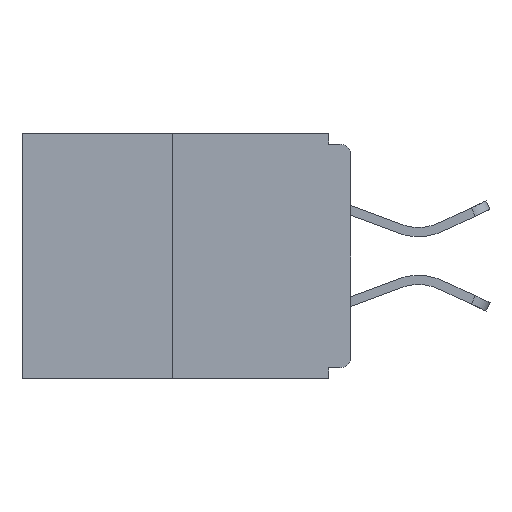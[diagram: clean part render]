
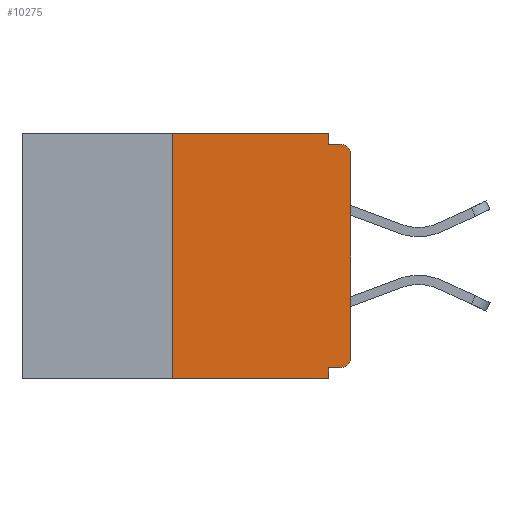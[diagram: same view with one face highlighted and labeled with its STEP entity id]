
A CAD part, left-side view. The second image highlights one B-rep face of the part: STEP entity #10275.
In plain terms, the highlighted planar face has unit normal (-1, 0, 0).
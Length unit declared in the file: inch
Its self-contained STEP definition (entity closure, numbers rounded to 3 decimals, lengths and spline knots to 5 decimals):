
#341 = VECTOR ( 'NONE', #5131, 39.37008 ) ;
#343 = VERTEX_POINT ( 'NONE', #4342 ) ;
#384 = LINE ( 'NONE', #3986, #11502 ) ;
#429 = LINE ( 'NONE', #2580, #6251 ) ;
#442 = CIRCLE ( 'NONE', #6177, 0.015 ) ;
#459 = LINE ( 'NONE', #3136, #7637 ) ;
#1343 = FACE_OUTER_BOUND ( 'NONE', #12251, .T. ) ;
#1357 = CARTESIAN_POINT ( 'NONE',  ( 0., 0.46, -0.343 ) ) ;
#1565 = DIRECTION ( 'NONE',  ( 0., 0., -1. ) ) ;
#1659 = VERTEX_POINT ( 'NONE', #4040 ) ;
#1890 = DIRECTION ( 'NONE',  ( 0., 0., -1. ) ) ;
#2443 = CARTESIAN_POINT ( 'NONE',  ( 0., 0.031, -0.015 ) ) ;
#2580 = CARTESIAN_POINT ( 'NONE',  ( 0., 0., 0. ) ) ;
#2655 = ORIENTED_EDGE ( 'NONE', *, *, #3611, .F. ) ;
#2685 = CARTESIAN_POINT ( 'NONE',  ( 0., 0.031, 0. ) ) ;
#2818 = CARTESIAN_POINT ( 'NONE',  ( 0., 0.015, -0.328 ) ) ;
#3136 = CARTESIAN_POINT ( 'NONE',  ( 0., 0.031, -0.343 ) ) ;
#3190 = VERTEX_POINT ( 'NONE', #12193 ) ;
#3315 = LINE ( 'NONE', #2685, #12921 ) ;
#3611 = EDGE_CURVE ( 'NONE', #18052, #10127, #8825, .T. ) ;
#3906 = DIRECTION ( 'NONE',  ( 0., 1., 0. ) ) ;
#3986 = CARTESIAN_POINT ( 'NONE',  ( 0., 0., -0.015 ) ) ;
#4040 = CARTESIAN_POINT ( 'NONE',  ( 0., 0.015, -0.015 ) ) ;
#4149 = CARTESIAN_POINT ( 'NONE',  ( 0., 0., -0.03 ) ) ;
#4192 = DIRECTION ( 'NONE',  ( -1., 0., 0. ) ) ;
#4341 = DIRECTION ( 'NONE',  ( 0., -1., 0. ) ) ;
#4342 = CARTESIAN_POINT ( 'NONE',  ( 0., 0., -0.313 ) ) ;
#4604 = VERTEX_POINT ( 'NONE', #4149 ) ;
#5131 = DIRECTION ( 'NONE',  ( 0., -1., 0. ) ) ;
#5533 = EDGE_CURVE ( 'NONE', #4604, #1659, #15086, .T. ) ;
#5534 = PLANE ( 'NONE',  #8655 ) ;
#6177 = AXIS2_PLACEMENT_3D ( 'NONE', #9018, #11947, #17567 ) ;
#6251 = VECTOR ( 'NONE', #6882, 39.37008 ) ;
#6738 = DIRECTION ( 'NONE',  ( 0., -1., 0. ) ) ;
#6882 = DIRECTION ( 'NONE',  ( 0., 0., 1. ) ) ;
#7225 = LINE ( 'NONE', #1357, #8545 ) ;
#7605 = VERTEX_POINT ( 'NONE', #2818 ) ;
#7637 = VECTOR ( 'NONE', #1890, 39.37008 ) ;
#7959 = DIRECTION ( 'NONE',  ( 0., 0., 1. ) ) ;
#8083 = ORIENTED_EDGE ( 'NONE', *, *, #5533, .T. ) ;
#8141 = CARTESIAN_POINT ( 'NONE',  ( 0., 0.25, 0. ) ) ;
#8416 = VERTEX_POINT ( 'NONE', #2443 ) ;
#8545 = VECTOR ( 'NONE', #4341, 39.37008 ) ;
#8655 = AXIS2_PLACEMENT_3D ( 'NONE', #15348, #16763, #9751 ) ;
#8825 = LINE ( 'NONE', #10651, #341 ) ;
#8838 = ORIENTED_EDGE ( 'NONE', *, *, #10258, .F. ) ;
#9018 = CARTESIAN_POINT ( 'NONE',  ( 0., 0.015, -0.313 ) ) ;
#9278 = ORIENTED_EDGE ( 'NONE', *, *, #9957, .T. ) ;
#9738 = VERTEX_POINT ( 'NONE', #16681 ) ;
#9751 = DIRECTION ( 'NONE',  ( 0., 0., -1. ) ) ;
#9957 = EDGE_CURVE ( 'NONE', #3190, #9738, #7225, .T. ) ;
#9963 = CARTESIAN_POINT ( 'NONE',  ( 0., 0.031, 0. ) ) ;
#10046 = VECTOR ( 'NONE', #7959, 39.37008 ) ;
#10127 = VERTEX_POINT ( 'NONE', #9963 ) ;
#10258 = EDGE_CURVE ( 'NONE', #10127, #8416, #3315, .T. ) ;
#10275 = ADVANCED_FACE ( 'NONE', ( #1343 ), #5534, .F. ) ;
#10527 = EDGE_CURVE ( 'NONE', #3190, #18052, #16642, .T. ) ;
#10601 = VECTOR ( 'NONE', #3906, 39.37008 ) ;
#10651 = CARTESIAN_POINT ( 'NONE',  ( 0., 0.46, 0. ) ) ;
#11271 = CARTESIAN_POINT ( 'NONE',  ( 0., 0.015, -0.03 ) ) ;
#11426 = AXIS2_PLACEMENT_3D ( 'NONE', #11271, #4192, #1565 ) ;
#11502 = VECTOR ( 'NONE', #6738, 39.37008 ) ;
#11673 = VERTEX_POINT ( 'NONE', #13190 ) ;
#11947 = DIRECTION ( 'NONE',  ( -1., 0., 0. ) ) ;
#12160 = EDGE_CURVE ( 'NONE', #7605, #343, #442, .T. ) ;
#12193 = CARTESIAN_POINT ( 'NONE',  ( 0., 0.25, -0.343 ) ) ;
#12251 = EDGE_LOOP ( 'NONE', ( #2655, #13289, #9278, #12424, #14771, #15233, #17931, #8083, #13475, #8838 ) ) ;
#12268 = CARTESIAN_POINT ( 'NONE',  ( 0., 0., -0.328 ) ) ;
#12424 = ORIENTED_EDGE ( 'NONE', *, *, #14399, .F. ) ;
#12921 = VECTOR ( 'NONE', #13925, 39.37008 ) ;
#13190 = CARTESIAN_POINT ( 'NONE',  ( 0., 0.031, -0.328 ) ) ;
#13289 = ORIENTED_EDGE ( 'NONE', *, *, #10527, .F. ) ;
#13475 = ORIENTED_EDGE ( 'NONE', *, *, #17724, .F. ) ;
#13925 = DIRECTION ( 'NONE',  ( 0., 0., -1. ) ) ;
#13960 = EDGE_CURVE ( 'NONE', #7605, #11673, #15650, .T. ) ;
#14399 = EDGE_CURVE ( 'NONE', #11673, #9738, #459, .T. ) ;
#14771 = ORIENTED_EDGE ( 'NONE', *, *, #13960, .F. ) ;
#15086 = CIRCLE ( 'NONE', #11426, 0.015 ) ;
#15233 = ORIENTED_EDGE ( 'NONE', *, *, #12160, .T. ) ;
#15348 = CARTESIAN_POINT ( 'NONE',  ( 0., 0.46, 0. ) ) ;
#15543 = EDGE_CURVE ( 'NONE', #343, #4604, #429, .T. ) ;
#15650 = LINE ( 'NONE', #12268, #10601 ) ;
#16257 = CARTESIAN_POINT ( 'NONE',  ( 0., 0.25, 0. ) ) ;
#16642 = LINE ( 'NONE', #8141, #10046 ) ;
#16681 = CARTESIAN_POINT ( 'NONE',  ( 0., 0.031, -0.343 ) ) ;
#16763 = DIRECTION ( 'NONE',  ( 1., 0., 0. ) ) ;
#17567 = DIRECTION ( 'NONE',  ( 0., 0., -1. ) ) ;
#17724 = EDGE_CURVE ( 'NONE', #8416, #1659, #384, .T. ) ;
#17931 = ORIENTED_EDGE ( 'NONE', *, *, #15543, .T. ) ;
#18052 = VERTEX_POINT ( 'NONE', #16257 ) ;
